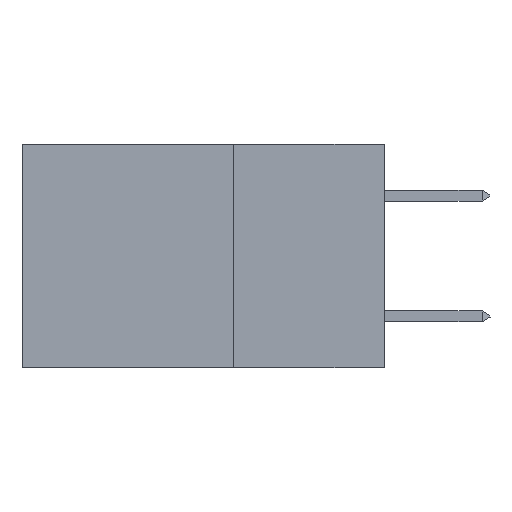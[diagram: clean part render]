
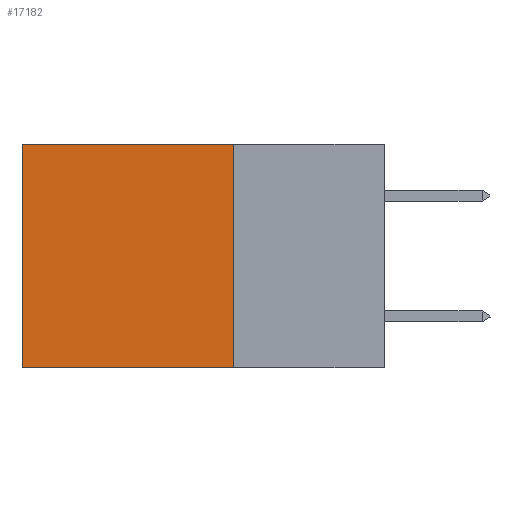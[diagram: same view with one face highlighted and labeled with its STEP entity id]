
A CAD part, left-side view. The second image highlights one B-rep face of the part: STEP entity #17182.
In plain terms, the highlighted planar face has unit normal (-1, 0, 0).
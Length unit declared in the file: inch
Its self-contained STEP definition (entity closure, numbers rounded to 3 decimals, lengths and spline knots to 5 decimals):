
#1050 = ORIENTED_EDGE ( 'NONE', *, *, #16705, .T. ) ;
#1327 = DIRECTION ( 'NONE',  ( 0., 0., -1. ) ) ;
#2012 = CARTESIAN_POINT ( 'NONE',  ( 0.2875, 0.6, 0. ) ) ;
#2231 = DIRECTION ( 'NONE',  ( 0., 1., 0. ) ) ;
#3394 = LINE ( 'NONE', #29296, #4230 ) ;
#3608 = PLANE ( 'NONE',  #7914 ) ;
#4124 = ORIENTED_EDGE ( 'NONE', *, *, #11487, .F. ) ;
#4230 = VECTOR ( 'NONE', #1327, 39.37008 ) ;
#4717 = EDGE_CURVE ( 'NONE', #31673, #5579, #31093, .T. ) ;
#5579 = VERTEX_POINT ( 'NONE', #29272 ) ;
#6692 = CARTESIAN_POINT ( 'NONE',  ( 0.2875, 0.25, 0. ) ) ;
#7914 = AXIS2_PLACEMENT_3D ( 'NONE', #26560, #15708, #15927 ) ;
#8090 = CARTESIAN_POINT ( 'NONE',  ( 0.2875, 0.25, 0. ) ) ;
#9146 = LINE ( 'NONE', #22533, #32692 ) ;
#9549 = EDGE_CURVE ( 'NONE', #31836, #5579, #9146, .T. ) ;
#10734 = DIRECTION ( 'NONE',  ( 0., 1., 0. ) ) ;
#10752 = VECTOR ( 'NONE', #10734, 39.37008 ) ;
#11487 = EDGE_CURVE ( 'NONE', #15823, #31836, #3394, .T. ) ;
#13478 = CARTESIAN_POINT ( 'NONE',  ( 0.2875, 0.25, -0.37 ) ) ;
#15708 = DIRECTION ( 'NONE',  ( 1., 0., 0. ) ) ;
#15823 = VERTEX_POINT ( 'NONE', #6692 ) ;
#15927 = DIRECTION ( 'NONE',  ( 0., 0., -1. ) ) ;
#16705 = EDGE_CURVE ( 'NONE', #15823, #31673, #24774, .T. ) ;
#17182 = ADVANCED_FACE ( 'NONE', ( #17918 ), #3608, .F. ) ;
#17918 = FACE_OUTER_BOUND ( 'NONE', #19877, .T. ) ;
#19877 = EDGE_LOOP ( 'NONE', ( #23287, #25448, #4124, #1050 ) ) ;
#20257 = CARTESIAN_POINT ( 'NONE',  ( 0.2875, 0.6, 0. ) ) ;
#21581 = VECTOR ( 'NONE', #32617, 39.37008 ) ;
#22533 = CARTESIAN_POINT ( 'NONE',  ( 0.2875, 0.25, -0.37 ) ) ;
#23287 = ORIENTED_EDGE ( 'NONE', *, *, #4717, .T. ) ;
#24774 = LINE ( 'NONE', #8090, #10752 ) ;
#25448 = ORIENTED_EDGE ( 'NONE', *, *, #9549, .F. ) ;
#26560 = CARTESIAN_POINT ( 'NONE',  ( 0.2875, 0.25, 0. ) ) ;
#29272 = CARTESIAN_POINT ( 'NONE',  ( 0.2875, 0.6, -0.37 ) ) ;
#29296 = CARTESIAN_POINT ( 'NONE',  ( 0.2875, 0.25, 0. ) ) ;
#31093 = LINE ( 'NONE', #2012, #21581 ) ;
#31673 = VERTEX_POINT ( 'NONE', #20257 ) ;
#31836 = VERTEX_POINT ( 'NONE', #13478 ) ;
#32617 = DIRECTION ( 'NONE',  ( 0., 0., -1. ) ) ;
#32692 = VECTOR ( 'NONE', #2231, 39.37008 ) ;
